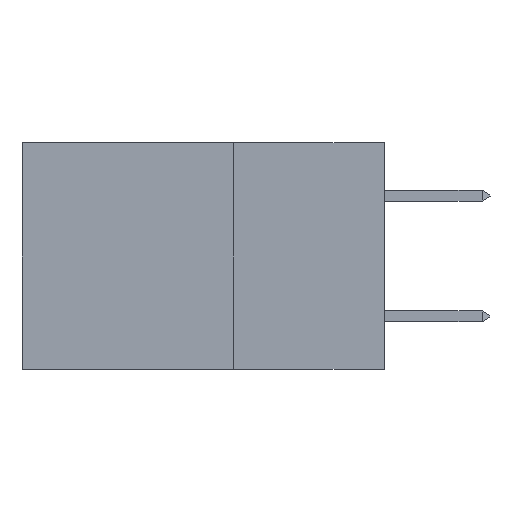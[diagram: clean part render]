
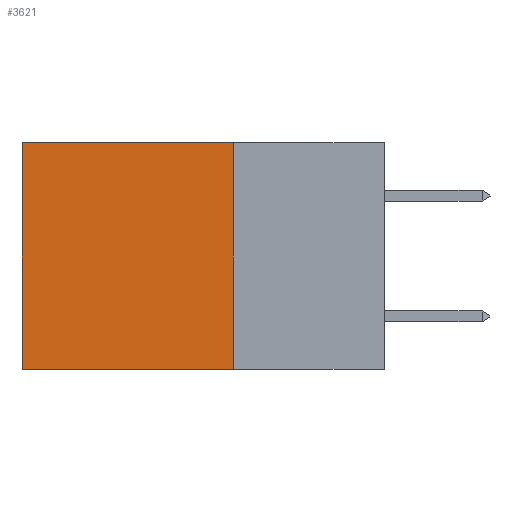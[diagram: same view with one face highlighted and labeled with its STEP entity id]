
A CAD part, left-side view. The second image highlights one B-rep face of the part: STEP entity #3621.
In plain terms, the highlighted planar face has unit normal (-1, 0, 0).
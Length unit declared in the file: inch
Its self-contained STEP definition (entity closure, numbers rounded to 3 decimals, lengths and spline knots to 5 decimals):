
#619 = EDGE_CURVE ( 'NONE', #6661, #1276, #5617, .T. ) ;
#853 = EDGE_CURVE ( 'NONE', #1276, #1242, #8245, .T. ) ;
#1129 = ORIENTED_EDGE ( 'NONE', *, *, #619, .T. ) ;
#1196 = CARTESIAN_POINT ( 'NONE',  ( 0.2875, 0.25, 0. ) ) ;
#1242 = VERTEX_POINT ( 'NONE', #2988 ) ;
#1276 = VERTEX_POINT ( 'NONE', #5190 ) ;
#1346 = DIRECTION ( 'NONE',  ( 0., 1., 0. ) ) ;
#1877 = VECTOR ( 'NONE', #7797, 39.37008 ) ;
#1960 = AXIS2_PLACEMENT_3D ( 'NONE', #2809, #4355, #9698 ) ;
#2020 = VECTOR ( 'NONE', #2839, 39.37008 ) ;
#2166 = FACE_OUTER_BOUND ( 'NONE', #2417, .T. ) ;
#2272 = VERTEX_POINT ( 'NONE', #5918 ) ;
#2417 = EDGE_LOOP ( 'NONE', ( #8961, #2896, #6871, #1129 ) ) ;
#2809 = CARTESIAN_POINT ( 'NONE',  ( 0.2875, 0.25, -0.375 ) ) ;
#2839 = DIRECTION ( 'NONE',  ( 0., 1., 0. ) ) ;
#2896 = ORIENTED_EDGE ( 'NONE', *, *, #6406, .F. ) ;
#2988 = CARTESIAN_POINT ( 'NONE',  ( 0.2875, 0.6, -0.375 ) ) ;
#3621 = ADVANCED_FACE ( 'NONE', ( #2166 ), #8210, .F. ) ;
#3904 = LINE ( 'NONE', #8913, #9696 ) ;
#4355 = DIRECTION ( 'NONE',  ( 1., 0., 0. ) ) ;
#4430 = VECTOR ( 'NONE', #9153, 39.37008 ) ;
#4589 = CARTESIAN_POINT ( 'NONE',  ( 0.2875, 0.25, -0.375 ) ) ;
#5190 = CARTESIAN_POINT ( 'NONE',  ( 0.2875, 0.6, 0. ) ) ;
#5318 = CARTESIAN_POINT ( 'NONE',  ( 0.2875, 0.6, -0.375 ) ) ;
#5617 = LINE ( 'NONE', #1196, #2020 ) ;
#5918 = CARTESIAN_POINT ( 'NONE',  ( 0.2875, 0.25, -0.375 ) ) ;
#6021 = EDGE_CURVE ( 'NONE', #6661, #2272, #6169, .T. ) ;
#6169 = LINE ( 'NONE', #4589, #1877 ) ;
#6406 = EDGE_CURVE ( 'NONE', #2272, #1242, #3904, .T. ) ;
#6661 = VERTEX_POINT ( 'NONE', #7709 ) ;
#6871 = ORIENTED_EDGE ( 'NONE', *, *, #6021, .F. ) ;
#7709 = CARTESIAN_POINT ( 'NONE',  ( 0.2875, 0.25, 0. ) ) ;
#7797 = DIRECTION ( 'NONE',  ( 0., 0., -1. ) ) ;
#8210 = PLANE ( 'NONE',  #1960 ) ;
#8245 = LINE ( 'NONE', #5318, #4430 ) ;
#8913 = CARTESIAN_POINT ( 'NONE',  ( 0.2875, 0.25, -0.375 ) ) ;
#8961 = ORIENTED_EDGE ( 'NONE', *, *, #853, .T. ) ;
#9153 = DIRECTION ( 'NONE',  ( 0., 0., -1. ) ) ;
#9696 = VECTOR ( 'NONE', #1346, 39.37008 ) ;
#9698 = DIRECTION ( 'NONE',  ( 0., 0., -1. ) ) ;
